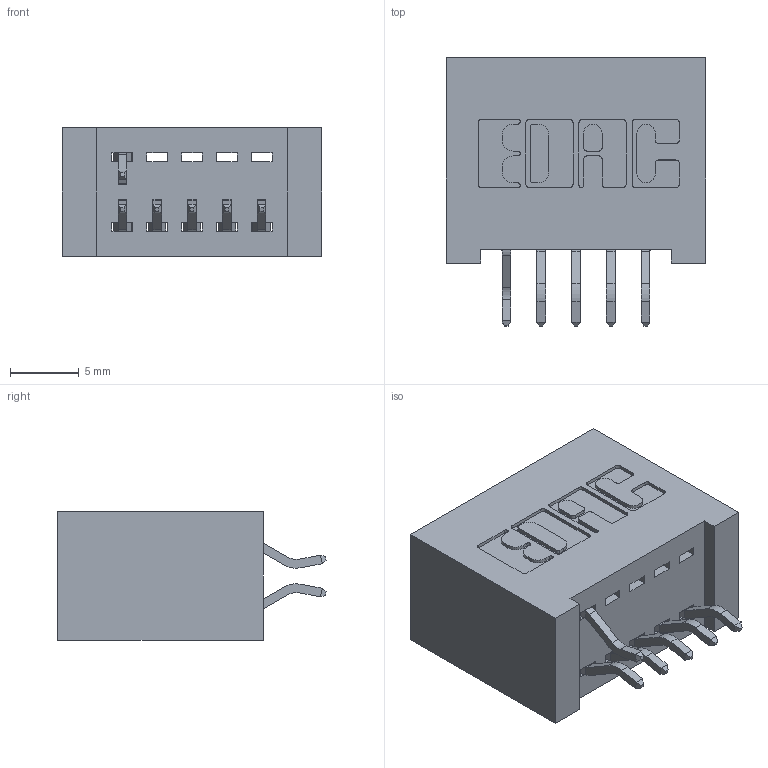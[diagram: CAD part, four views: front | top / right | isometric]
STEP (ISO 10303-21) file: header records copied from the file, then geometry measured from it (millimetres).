
FILE_DESCRIPTION (( 'STEP AP203' ), '1' );
FILE_NAME ('342-010-556-201.STEP', '2018-08-10T13:55:36', ( '' ), ( '' ), 'SwSTEP 2.0', 'SolidWorks 2016', '' );
FILE_SCHEMA (( 'CONFIG_CONTROL_DESIGN' ));
Length unit declared in the file: inch
Products named in the file (3): 342 Part_Lugless; 345-292-001_556 Tail; 342-010-556-201
Assembly tree (7 placements, depth 2):
  342-010-556-201
    342 Part_Lugless
    345-292-001_556 Tail  x6
Bounding box: 18.95 x 19.58 x 9.4 mm (x, y, z)
Volume: 1930.7 mm3; surface area: 2472.5 mm2
Topology: 7 solids, 7 shells, 474 faces, 1397 edges, 922 vertices
Faces by surface type: plane 326, cylinder 148
Entity records: 7685 total; most frequent: CARTESIAN_POINT 1346, ORIENTED_EDGE 1274, DIRECTION 1193, EDGE_CURVE 637, VECTOR 509, LINE 509, VERTEX_POINT 422, AXIS2_PLACEMENT_3D 342
